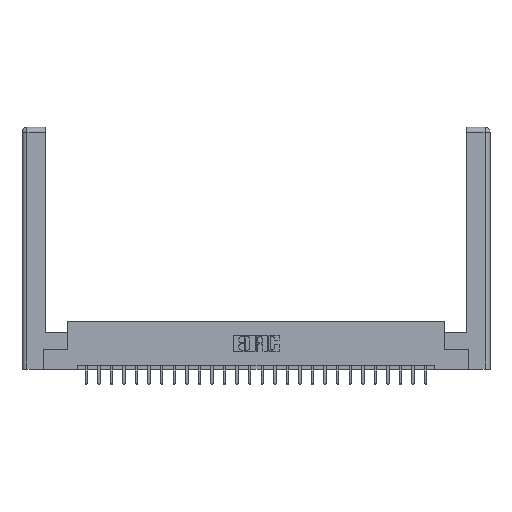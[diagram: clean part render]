
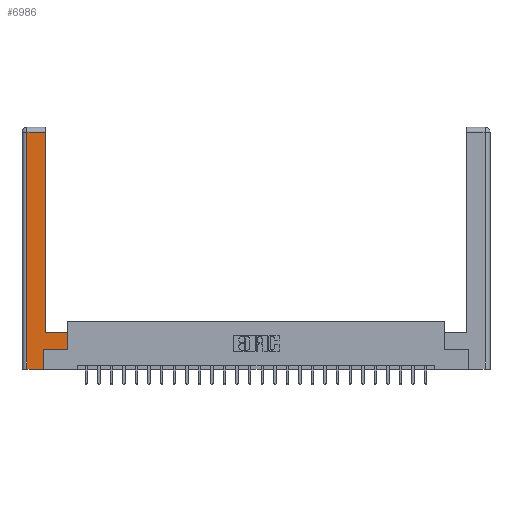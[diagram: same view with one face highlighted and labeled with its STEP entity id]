
A CAD part, top view. The second image highlights one B-rep face of the part: STEP entity #6986.
In plain terms, the highlighted planar face has unit normal (0, 0, 1).
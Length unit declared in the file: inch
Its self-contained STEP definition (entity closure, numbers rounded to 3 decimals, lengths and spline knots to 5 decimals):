
#10 = VECTOR ( 'NONE', #10708, 39.37008 ) ;
#201 = CARTESIAN_POINT ( 'NONE',  ( 0.0615, 2.94, 0. ) ) ;
#352 = EDGE_CURVE ( 'NONE', #21501, #10995, #1510, .T. ) ;
#360 = VECTOR ( 'NONE', #14966, 39.37008 ) ;
#722 = LINE ( 'NONE', #26042, #21705 ) ;
#851 = VECTOR ( 'NONE', #4211, 39.37008 ) ;
#1074 = EDGE_CURVE ( 'NONE', #2415, #5066, #24350, .T. ) ;
#1174 = PLANE ( 'NONE',  #6726 ) ;
#1510 = LINE ( 'NONE', #201, #13579 ) ;
#1711 = DIRECTION ( 'NONE',  ( 0., 1., 0. ) ) ;
#1929 = ORIENTED_EDGE ( 'NONE', *, *, #7312, .T. ) ;
#2415 = VERTEX_POINT ( 'NONE', #18350 ) ;
#3390 = LINE ( 'NONE', #19462, #13547 ) ;
#3522 = ORIENTED_EDGE ( 'NONE', *, *, #7643, .T. ) ;
#3932 = VERTEX_POINT ( 'NONE', #6361 ) ;
#4211 = DIRECTION ( 'NONE',  ( 1., 0., 0. ) ) ;
#4238 = CARTESIAN_POINT ( 'NONE',  ( 0.265, 0., 0. ) ) ;
#5023 = ORIENTED_EDGE ( 'NONE', *, *, #12195, .T. ) ;
#5066 = VERTEX_POINT ( 'NONE', #15293 ) ;
#5409 = VERTEX_POINT ( 'NONE', #18275 ) ;
#5750 = LINE ( 'NONE', #25355, #360 ) ;
#6361 = CARTESIAN_POINT ( 'NONE',  ( 0.565, 0.45, 0. ) ) ;
#6601 = ORIENTED_EDGE ( 'NONE', *, *, #14185, .T. ) ;
#6726 = AXIS2_PLACEMENT_3D ( 'NONE', #11358, #15469, #19288 ) ;
#6845 = ORIENTED_EDGE ( 'NONE', *, *, #24740, .T. ) ;
#6986 = ADVANCED_FACE ( 'NONE', ( #15581 ), #1174, .F. ) ;
#7187 = VECTOR ( 'NONE', #10692, 39.37008 ) ;
#7312 = EDGE_CURVE ( 'NONE', #12775, #21501, #10127, .T. ) ;
#7643 = EDGE_CURVE ( 'NONE', #3932, #12775, #23785, .T. ) ;
#9147 = VECTOR ( 'NONE', #17630, 39.37008 ) ;
#9693 = VERTEX_POINT ( 'NONE', #11403 ) ;
#10127 = LINE ( 'NONE', #20858, #10 ) ;
#10692 = DIRECTION ( 'NONE',  ( 1., 0., 0. ) ) ;
#10708 = DIRECTION ( 'NONE',  ( 0., 1., 0. ) ) ;
#10945 = ORIENTED_EDGE ( 'NONE', *, *, #352, .T. ) ;
#10995 = VERTEX_POINT ( 'NONE', #11923 ) ;
#11358 = CARTESIAN_POINT ( 'NONE',  ( 0., 0., 0. ) ) ;
#11403 = CARTESIAN_POINT ( 'NONE',  ( 0.565, 0.245, 0. ) ) ;
#11923 = CARTESIAN_POINT ( 'NONE',  ( 0.0615, 2.94, 0. ) ) ;
#12195 = EDGE_CURVE ( 'NONE', #5066, #5409, #5750, .T. ) ;
#12309 = EDGE_LOOP ( 'NONE', ( #1929, #10945, #6601, #16691, #5023, #13168, #6845, #3522 ) ) ;
#12775 = VERTEX_POINT ( 'NONE', #16718 ) ;
#12777 = DIRECTION ( 'NONE',  ( -1., 0., 0. ) ) ;
#13168 = ORIENTED_EDGE ( 'NONE', *, *, #18594, .T. ) ;
#13302 = DIRECTION ( 'NONE',  ( 0., -1., 0. ) ) ;
#13547 = VECTOR ( 'NONE', #13302, 39.37008 ) ;
#13579 = VECTOR ( 'NONE', #12777, 39.37008 ) ;
#14051 = CARTESIAN_POINT ( 'NONE',  ( 0.295, 2.94, 0. ) ) ;
#14185 = EDGE_CURVE ( 'NONE', #10995, #2415, #3390, .T. ) ;
#14966 = DIRECTION ( 'NONE',  ( 0., 1., 0. ) ) ;
#15293 = CARTESIAN_POINT ( 'NONE',  ( 0.265, 0., 0. ) ) ;
#15469 = DIRECTION ( 'NONE',  ( 0., 0., -1. ) ) ;
#15581 = FACE_OUTER_BOUND ( 'NONE', #12309, .T. ) ;
#16691 = ORIENTED_EDGE ( 'NONE', *, *, #1074, .T. ) ;
#16718 = CARTESIAN_POINT ( 'NONE',  ( 0.295, 0.45, 0. ) ) ;
#17630 = DIRECTION ( 'NONE',  ( -1., 0., 0. ) ) ;
#18275 = CARTESIAN_POINT ( 'NONE',  ( 0.265, 0.245, 0. ) ) ;
#18350 = CARTESIAN_POINT ( 'NONE',  ( 0.0615, 0., 0. ) ) ;
#18594 = EDGE_CURVE ( 'NONE', #5409, #9693, #24372, .T. ) ;
#19288 = DIRECTION ( 'NONE',  ( -1., 0., 0. ) ) ;
#19462 = CARTESIAN_POINT ( 'NONE',  ( 0.0615, 0., 0. ) ) ;
#20858 = CARTESIAN_POINT ( 'NONE',  ( 0.295, 3., 0. ) ) ;
#21501 = VERTEX_POINT ( 'NONE', #14051 ) ;
#21705 = VECTOR ( 'NONE', #1711, 39.37008 ) ;
#22435 = CARTESIAN_POINT ( 'NONE',  ( 0.565, 0.245, 0. ) ) ;
#23694 = CARTESIAN_POINT ( 'NONE',  ( 0.295, 0.45, 0. ) ) ;
#23785 = LINE ( 'NONE', #23694, #9147 ) ;
#24350 = LINE ( 'NONE', #4238, #7187 ) ;
#24372 = LINE ( 'NONE', #22435, #851 ) ;
#24740 = EDGE_CURVE ( 'NONE', #9693, #3932, #722, .T. ) ;
#25355 = CARTESIAN_POINT ( 'NONE',  ( 0.265, 0.245, 0. ) ) ;
#26042 = CARTESIAN_POINT ( 'NONE',  ( 0.565, 0.45, 0. ) ) ;
